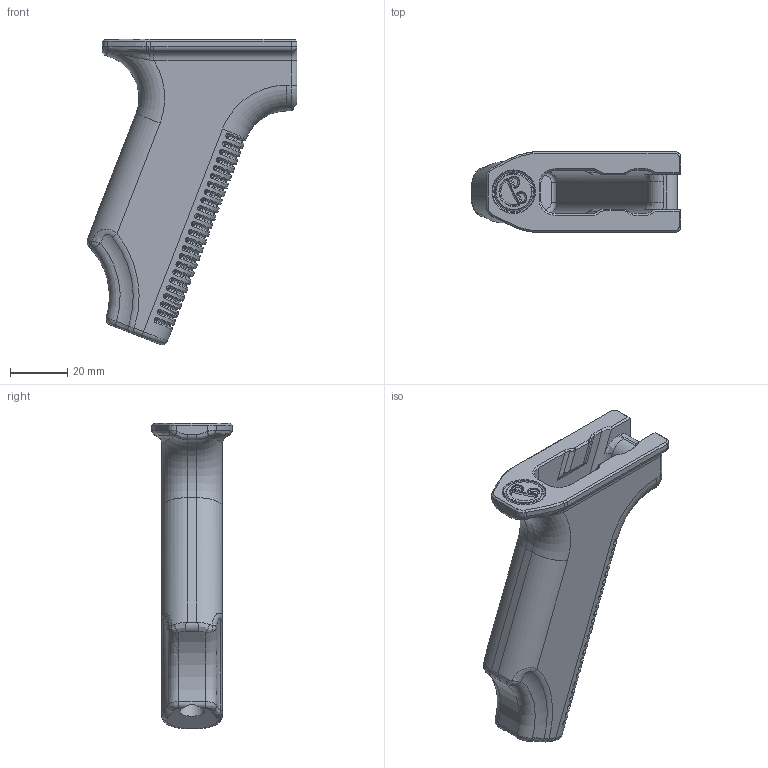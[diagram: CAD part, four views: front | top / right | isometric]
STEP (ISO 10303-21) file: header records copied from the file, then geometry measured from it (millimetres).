
FILE_DESCRIPTION(/* description */ (''),/* implementation_level */ '2;1');
FILE_NAME(/* name */ '3FTech Cutback Grip.step',/* time_stamp */ '2021-09-12T08:32:18-04:00',/* author */ (''),/* organization */ (''),/* preprocessor_version */ 'ST-DEVELOPER v18.1',/* originating_system */ 'Autodesk Translation Framework v10.10.0.1391',/* authorisation */ '');
FILE_SCHEMA (('AUTOMOTIVE_DESIGN { 1 0 10303 214 3 1 1 }'));
Length unit declared in the file: millimetre
Products named in the file (1): 3FTech Cutback Grip
Bounding box: 73.19 x 28 x 106.55 mm (x, y, z)
Volume: 43577.6 mm3; surface area: 23000.2 mm2
Topology: 1 solids, 1 shells, 829 faces, 1940 edges, 1108 vertices
Faces by surface type: cylinder 259, torus 224, bspline 184, plane 140, cone 18, sphere 4
Full cylindrical faces by diameter (mm): 6 x1, 8.8 x1, 12.778 x1, 14.758 x1
Entity records: 30805 total; most frequent: CARTESIAN_POINT 12558, ORIENTED_EDGE 3860, DIRECTION 3836, EDGE_CURVE 1930, AXIS2_PLACEMENT_3D 1625, VERTEX_POINT 1108, CIRCLE 973, EDGE_LOOP 836
